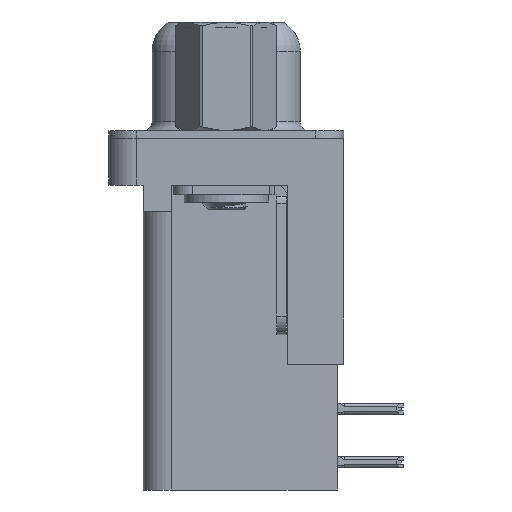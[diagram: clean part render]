
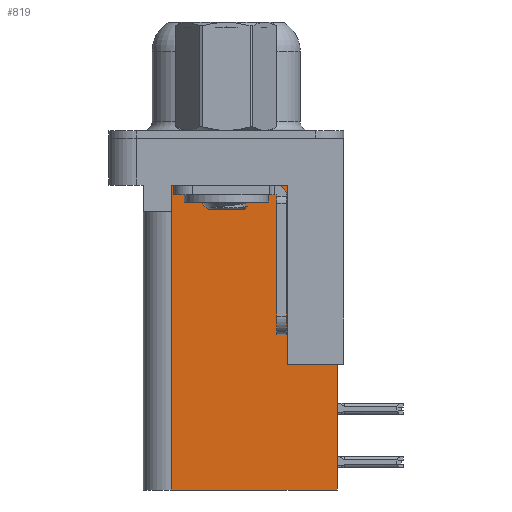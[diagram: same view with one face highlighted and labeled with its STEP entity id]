
A CAD part, left-side view. The second image highlights one B-rep face of the part: STEP entity #819.
In plain terms, the highlighted planar face has unit normal (-1, 0, 0).
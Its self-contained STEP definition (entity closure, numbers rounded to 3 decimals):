
#192 = DIRECTION ( 'NONE',  ( 0., 0., 1. ) ) ;
#232 = VECTOR ( 'NONE', #6287, 1000. ) ;
#415 = FACE_OUTER_BOUND ( 'NONE', #24396, .T. ) ;
#422 = CARTESIAN_POINT ( 'NONE',  ( 3.79, -5.925, -18.76 ) ) ;
#455 = LINE ( 'NONE', #19654, #232 ) ;
#819 = ADVANCED_FACE ( 'NONE', ( #415 ), #4348, .F. ) ;
#842 = VECTOR ( 'NONE', #25582, 1000. ) ;
#868 = LINE ( 'NONE', #12034, #842 ) ;
#1114 = CARTESIAN_POINT ( 'NONE',  ( 3.79, -3.295, -18.76 ) ) ;
#1425 = AXIS2_PLACEMENT_3D ( 'NONE', #7219, #7086, #27571 ) ;
#1492 = CARTESIAN_POINT ( 'NONE',  ( 3.79, -3.295, -2.5 ) ) ;
#1711 = CARTESIAN_POINT ( 'NONE',  ( 3.79, 2.925, -18.76 ) ) ;
#2483 = CARTESIAN_POINT ( 'NONE',  ( 3.79, 2.925, -18.76 ) ) ;
#2551 = ORIENTED_EDGE ( 'NONE', *, *, #11989, .F. ) ;
#2933 = ORIENTED_EDGE ( 'NONE', *, *, #5906, .T. ) ;
#4246 = VERTEX_POINT ( 'NONE', #1711 ) ;
#4348 = PLANE ( 'NONE',  #1425 ) ;
#4711 = DIRECTION ( 'NONE',  ( 0., 0., 1. ) ) ;
#4740 = ORIENTED_EDGE ( 'NONE', *, *, #26568, .F. ) ;
#5165 = CARTESIAN_POINT ( 'NONE',  ( 3.79, 2.895, -3.9 ) ) ;
#5558 = VERTEX_POINT ( 'NONE', #13216 ) ;
#5906 = EDGE_CURVE ( 'NONE', #13017, #26270, #10110, .T. ) ;
#6006 = ORIENTED_EDGE ( 'NONE', *, *, #23640, .T. ) ;
#6287 = DIRECTION ( 'NONE',  ( 0., 0., -1. ) ) ;
#7086 = DIRECTION ( 'NONE',  ( 1., 0., 0. ) ) ;
#7219 = CARTESIAN_POINT ( 'NONE',  ( 3.79, -3.295, -18.76 ) ) ;
#7777 = VERTEX_POINT ( 'NONE', #5165 ) ;
#8420 = VERTEX_POINT ( 'NONE', #20951 ) ;
#9496 = VERTEX_POINT ( 'NONE', #422 ) ;
#9690 = VECTOR ( 'NONE', #10337, 1000. ) ;
#10032 = LINE ( 'NONE', #1492, #9690 ) ;
#10054 = VECTOR ( 'NONE', #192, 1000. ) ;
#10110 = LINE ( 'NONE', #1114, #10054 ) ;
#10337 = DIRECTION ( 'NONE',  ( 0., 1., 0. ) ) ;
#10426 = EDGE_CURVE ( 'NONE', #5558, #13017, #21470, .T. ) ;
#10743 = VECTOR ( 'NONE', #27054, 1000. ) ;
#10900 = LINE ( 'NONE', #24876, #10743 ) ;
#11925 = CARTESIAN_POINT ( 'NONE',  ( 3.79, -6.295, -12.05 ) ) ;
#11989 = EDGE_CURVE ( 'NONE', #4246, #8420, #16382, .T. ) ;
#12034 = CARTESIAN_POINT ( 'NONE',  ( 3.79, -3.295, -18.76 ) ) ;
#13017 = VERTEX_POINT ( 'NONE', #13250 ) ;
#13216 = CARTESIAN_POINT ( 'NONE',  ( 3.79, -5.925, -12.05 ) ) ;
#13250 = CARTESIAN_POINT ( 'NONE',  ( 3.79, -3.295, -12.05 ) ) ;
#13272 = ORIENTED_EDGE ( 'NONE', *, *, #26773, .F. ) ;
#14738 = ORIENTED_EDGE ( 'NONE', *, *, #10426, .T. ) ;
#16334 = VECTOR ( 'NONE', #4711, 1000. ) ;
#16382 = LINE ( 'NONE', #2483, #16334 ) ;
#16460 = DIRECTION ( 'NONE',  ( 0., 1., 0. ) ) ;
#16838 = CARTESIAN_POINT ( 'NONE',  ( 3.79, 0., -3.9 ) ) ;
#18462 = EDGE_CURVE ( 'NONE', #7777, #8420, #27587, .T. ) ;
#19121 = DIRECTION ( 'NONE',  ( 0., 1., 0. ) ) ;
#19654 = CARTESIAN_POINT ( 'NONE',  ( 3.79, -5.925, -2. ) ) ;
#20700 = CARTESIAN_POINT ( 'NONE',  ( 3.79, 2.895, -2.5 ) ) ;
#20951 = CARTESIAN_POINT ( 'NONE',  ( 3.79, 2.925, -3.9 ) ) ;
#21391 = VECTOR ( 'NONE', #16460, 1000. ) ;
#21470 = LINE ( 'NONE', #11925, #21391 ) ;
#22238 = CARTESIAN_POINT ( 'NONE',  ( 3.79, -3.295, -2.5 ) ) ;
#22304 = VERTEX_POINT ( 'NONE', #20700 ) ;
#23094 = ORIENTED_EDGE ( 'NONE', *, *, #23958, .T. ) ;
#23640 = EDGE_CURVE ( 'NONE', #22304, #7777, #10900, .T. ) ;
#23958 = EDGE_CURVE ( 'NONE', #26270, #22304, #10032, .T. ) ;
#24396 = EDGE_LOOP ( 'NONE', ( #23094, #6006, #28509, #2551, #4740, #13272, #14738, #2933 ) ) ;
#24876 = CARTESIAN_POINT ( 'NONE',  ( 3.79, 2.895, -3.9 ) ) ;
#25582 = DIRECTION ( 'NONE',  ( 0., 1., 0. ) ) ;
#26270 = VERTEX_POINT ( 'NONE', #22238 ) ;
#26568 = EDGE_CURVE ( 'NONE', #9496, #4246, #868, .T. ) ;
#26773 = EDGE_CURVE ( 'NONE', #5558, #9496, #455, .T. ) ;
#27054 = DIRECTION ( 'NONE',  ( 0., 0., -1. ) ) ;
#27205 = VECTOR ( 'NONE', #19121, 1000. ) ;
#27571 = DIRECTION ( 'NONE',  ( 0., 1., 0. ) ) ;
#27587 = LINE ( 'NONE', #16838, #27205 ) ;
#28509 = ORIENTED_EDGE ( 'NONE', *, *, #18462, .T. ) ;
